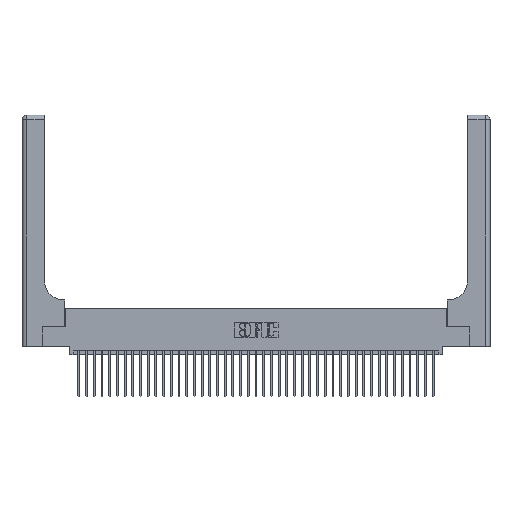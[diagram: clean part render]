
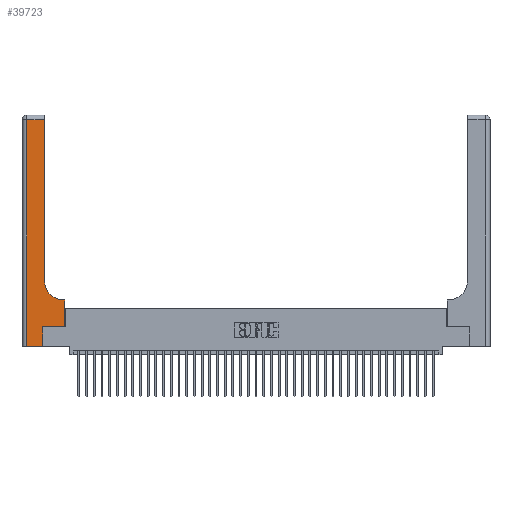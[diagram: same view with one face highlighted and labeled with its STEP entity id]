
A CAD part, top view. The second image highlights one B-rep face of the part: STEP entity #39723.
In plain terms, the highlighted planar face has unit normal (0, 0, 1).
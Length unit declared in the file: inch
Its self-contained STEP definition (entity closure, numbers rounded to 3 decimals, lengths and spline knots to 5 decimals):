
#446 = EDGE_CURVE ( 'NONE', #3319, #40566, #37210, .T. ) ;
#1541 = VECTOR ( 'NONE', #22960, 39.37008 ) ;
#2470 = EDGE_LOOP ( 'NONE', ( #9304, #9340, #10010, #10755, #11852, #13331, #13408, #13545, #13620 ) ) ;
#3172 = VERTEX_POINT ( 'NONE', #13939 ) ;
#3319 = VERTEX_POINT ( 'NONE', #27444 ) ;
#4900 = AXIS2_PLACEMENT_3D ( 'NONE', #35899, #16628, #39102 ) ;
#6281 = EDGE_CURVE ( 'NONE', #17188, #3172, #21170, .T. ) ;
#6824 = CARTESIAN_POINT ( 'NONE',  ( 0., 2.94, 0.37 ) ) ;
#7578 = FACE_OUTER_BOUND ( 'NONE', #2470, .T. ) ;
#8381 = DIRECTION ( 'NONE',  ( 0., 1., 0. ) ) ;
#9304 = ORIENTED_EDGE ( 'NONE', *, *, #6281, .T. ) ;
#9340 = ORIENTED_EDGE ( 'NONE', *, *, #17519, .T. ) ;
#9407 = LINE ( 'NONE', #27580, #34097 ) ;
#9919 = EDGE_CURVE ( 'NONE', #41478, #13877, #9407, .T. ) ;
#10010 = ORIENTED_EDGE ( 'NONE', *, *, #31328, .T. ) ;
#10054 = LINE ( 'NONE', #6824, #1541 ) ;
#10517 = VERTEX_POINT ( 'NONE', #40085 ) ;
#10755 = ORIENTED_EDGE ( 'NONE', *, *, #446, .T. ) ;
#11051 = VECTOR ( 'NONE', #39174, 39.37008 ) ;
#11778 = CARTESIAN_POINT ( 'NONE',  ( 0.269, 0.25, 0.37 ) ) ;
#11852 = ORIENTED_EDGE ( 'NONE', *, *, #24348, .T. ) ;
#13331 = ORIENTED_EDGE ( 'NONE', *, *, #17204, .T. ) ;
#13408 = ORIENTED_EDGE ( 'NONE', *, *, #27612, .T. ) ;
#13545 = ORIENTED_EDGE ( 'NONE', *, *, #9919, .T. ) ;
#13588 = VECTOR ( 'NONE', #34293, 39.37008 ) ;
#13620 = ORIENTED_EDGE ( 'NONE', *, *, #16177, .T. ) ;
#13672 = VECTOR ( 'NONE', #8381, 39.37008 ) ;
#13877 = VERTEX_POINT ( 'NONE', #19670 ) ;
#13939 = CARTESIAN_POINT ( 'NONE',  ( 0.2915, 2.94, 0.37 ) ) ;
#15086 = AXIS2_PLACEMENT_3D ( 'NONE', #36613, #17309, #39783 ) ;
#16177 = EDGE_CURVE ( 'NONE', #13877, #17188, #23645, .T. ) ;
#16628 = DIRECTION ( 'NONE',  ( 0., 0., -1. ) ) ;
#16702 = CARTESIAN_POINT ( 'NONE',  ( 0.269, 0., 0.37 ) ) ;
#17188 = VERTEX_POINT ( 'NONE', #37347 ) ;
#17204 = EDGE_CURVE ( 'NONE', #31354, #23244, #30732, .T. ) ;
#17309 = DIRECTION ( 'NONE',  ( 0., 0., -1. ) ) ;
#17519 = EDGE_CURVE ( 'NONE', #3172, #10517, #10054, .T. ) ;
#19403 = LINE ( 'NONE', #24746, #25988 ) ;
#19670 = CARTESIAN_POINT ( 'NONE',  ( 0.5415, 0.6, 0.37 ) ) ;
#21077 = VECTOR ( 'NONE', #31669, 39.37008 ) ;
#21170 = LINE ( 'NONE', #27652, #13672 ) ;
#21513 = DIRECTION ( 'NONE',  ( 0., 1., 0. ) ) ;
#22831 = VECTOR ( 'NONE', #29425, 39.37008 ) ;
#22960 = DIRECTION ( 'NONE',  ( -1., 0., 0. ) ) ;
#23244 = VERTEX_POINT ( 'NONE', #36909 ) ;
#23645 = CIRCLE ( 'NONE', #15086, 0.25 ) ;
#23847 = LINE ( 'NONE', #35838, #22831 ) ;
#24348 = EDGE_CURVE ( 'NONE', #40566, #31354, #35652, .T. ) ;
#24746 = CARTESIAN_POINT ( 'NONE',  ( 0.5585, 0.25, 0.37 ) ) ;
#25805 = CARTESIAN_POINT ( 'NONE',  ( 0.5585, 0.6, 0.37 ) ) ;
#25988 = VECTOR ( 'NONE', #21513, 39.37008 ) ;
#26217 = PLANE ( 'NONE',  #4900 ) ;
#27444 = CARTESIAN_POINT ( 'NONE',  ( 0.06, 0., 0.37 ) ) ;
#27580 = CARTESIAN_POINT ( 'NONE',  ( 0.2915, 0.6, 0.37 ) ) ;
#27612 = EDGE_CURVE ( 'NONE', #23244, #41478, #19403, .T. ) ;
#27652 = CARTESIAN_POINT ( 'NONE',  ( 0.2915, 3., 0.37 ) ) ;
#29425 = DIRECTION ( 'NONE',  ( 0., -1., 0. ) ) ;
#29566 = CARTESIAN_POINT ( 'NONE',  ( 0.269, 0.25, 0.37 ) ) ;
#30732 = LINE ( 'NONE', #11778, #13588 ) ;
#31328 = EDGE_CURVE ( 'NONE', #10517, #3319, #23847, .T. ) ;
#31354 = VERTEX_POINT ( 'NONE', #29566 ) ;
#31669 = DIRECTION ( 'NONE',  ( 1., 0., 0. ) ) ;
#33653 = CARTESIAN_POINT ( 'NONE',  ( 0.269, 0., 0.37 ) ) ;
#34097 = VECTOR ( 'NONE', #37240, 39.37008 ) ;
#34293 = DIRECTION ( 'NONE',  ( 1., 0., 0. ) ) ;
#34865 = CARTESIAN_POINT ( 'NONE',  ( 0., 0., 0.37 ) ) ;
#35652 = LINE ( 'NONE', #16702, #11051 ) ;
#35838 = CARTESIAN_POINT ( 'NONE',  ( 0.06, 3., 0.37 ) ) ;
#35899 = CARTESIAN_POINT ( 'NONE',  ( 0., 3., 0.37 ) ) ;
#36613 = CARTESIAN_POINT ( 'NONE',  ( 0.5415, 0.85, 0.37 ) ) ;
#36909 = CARTESIAN_POINT ( 'NONE',  ( 0.5585, 0.25, 0.37 ) ) ;
#37210 = LINE ( 'NONE', #34865, #21077 ) ;
#37240 = DIRECTION ( 'NONE',  ( -1., 0., 0. ) ) ;
#37347 = CARTESIAN_POINT ( 'NONE',  ( 0.2915, 0.85, 0.37 ) ) ;
#39102 = DIRECTION ( 'NONE',  ( -1., 0., 0. ) ) ;
#39174 = DIRECTION ( 'NONE',  ( 0., 1., 0. ) ) ;
#39723 = ADVANCED_FACE ( 'NONE', ( #7578 ), #26217, .F. ) ;
#39783 = DIRECTION ( 'NONE',  ( 1., 0., 0. ) ) ;
#40085 = CARTESIAN_POINT ( 'NONE',  ( 0.06, 2.94, 0.37 ) ) ;
#40566 = VERTEX_POINT ( 'NONE', #33653 ) ;
#41478 = VERTEX_POINT ( 'NONE', #25805 ) ;
